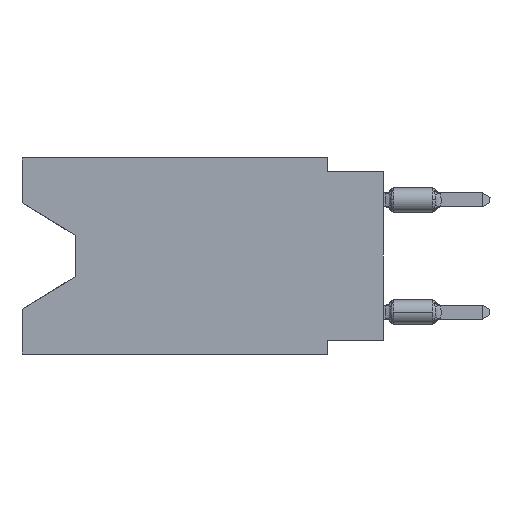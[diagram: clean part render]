
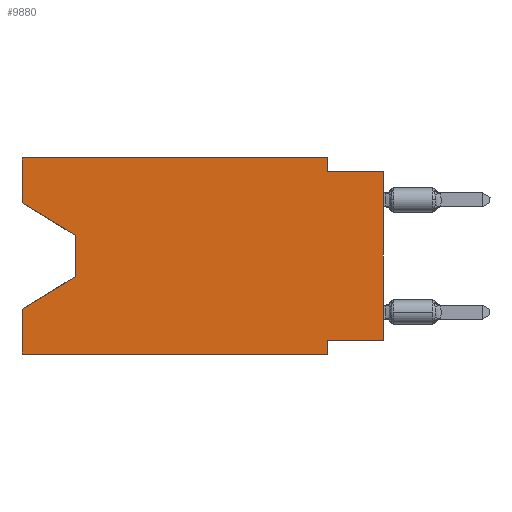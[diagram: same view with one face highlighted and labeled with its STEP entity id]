
A CAD part, left-side view. The second image highlights one B-rep face of the part: STEP entity #9880.
In plain terms, the highlighted planar face has unit normal (-1, 0, 0).
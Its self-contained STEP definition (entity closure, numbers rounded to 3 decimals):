
#218 = ORIENTED_EDGE ( 'NONE', *, *, #61031, .T. ) ;
#898 = LINE ( 'NONE', #48682, #18577 ) ;
#3849 = VERTEX_POINT ( 'NONE', #51764 ) ;
#3941 = CARTESIAN_POINT ( 'NONE',  ( 0., 13.97, -5.385 ) ) ;
#5513 = EDGE_CURVE ( 'NONE', #23257, #10101, #52324, .T. ) ;
#5767 = EDGE_CURVE ( 'NONE', #45476, #48817, #41096, .T. ) ;
#7909 = EDGE_CURVE ( 'NONE', #26975, #51505, #39138, .T. ) ;
#8350 = ORIENTED_EDGE ( 'NONE', *, *, #55840, .F. ) ;
#8451 = DIRECTION ( 'NONE',  ( 1., 0., 0. ) ) ;
#8663 = CARTESIAN_POINT ( 'NONE',  ( 0., 16.383, 0. ) ) ;
#8837 = CARTESIAN_POINT ( 'NONE',  ( 0., 16.383, 0. ) ) ;
#9020 = VECTOR ( 'NONE', #38017, 1000. ) ;
#9143 = DIRECTION ( 'NONE',  ( 0., -0.855, -0.519 ) ) ;
#9880 = ADVANCED_FACE ( 'NONE', ( #23721 ), #57855, .F. ) ;
#10101 = VERTEX_POINT ( 'NONE', #12437 ) ;
#10320 = LINE ( 'NONE', #8837, #57527 ) ;
#10482 = EDGE_LOOP ( 'NONE', ( #36207, #53071, #25910, #8350, #218, #14693, #40935, #35727, #20736, #42518, #43916, #48797 ) ) ;
#10778 = DIRECTION ( 'NONE',  ( 0., -1., 0. ) ) ;
#10949 = CARTESIAN_POINT ( 'NONE',  ( 0., 13.97, -5.385 ) ) ;
#11733 = VERTEX_POINT ( 'NONE', #34187 ) ;
#12019 = CARTESIAN_POINT ( 'NONE',  ( 0., 2.54, -8.89 ) ) ;
#12437 = CARTESIAN_POINT ( 'NONE',  ( 0., 16.383, 0. ) ) ;
#13182 = VECTOR ( 'NONE', #48444, 1000. ) ;
#14693 = ORIENTED_EDGE ( 'NONE', *, *, #51194, .F. ) ;
#15480 = VECTOR ( 'NONE', #26357, 1000. ) ;
#16600 = CARTESIAN_POINT ( 'NONE',  ( 0., 16.383, -8.89 ) ) ;
#17453 = VERTEX_POINT ( 'NONE', #34656 ) ;
#17732 = LINE ( 'NONE', #62361, #24379 ) ;
#17740 = VECTOR ( 'NONE', #61946, 1000. ) ;
#18225 = CARTESIAN_POINT ( 'NONE',  ( 0., 2.54, 0. ) ) ;
#18577 = VECTOR ( 'NONE', #33699, 1000. ) ;
#18623 = DIRECTION ( 'NONE',  ( 0., 0., -1. ) ) ;
#20293 = EDGE_CURVE ( 'NONE', #11733, #17453, #53243, .T. ) ;
#20736 = ORIENTED_EDGE ( 'NONE', *, *, #7909, .F. ) ;
#21251 = CARTESIAN_POINT ( 'NONE',  ( 0., 0., 0. ) ) ;
#21344 = DIRECTION ( 'NONE',  ( 0., 0., -1. ) ) ;
#21883 = LINE ( 'NONE', #21251, #15480 ) ;
#22812 = VERTEX_POINT ( 'NONE', #16600 ) ;
#23257 = VERTEX_POINT ( 'NONE', #51132 ) ;
#23378 = LINE ( 'NONE', #62272, #9020 ) ;
#23721 = FACE_OUTER_BOUND ( 'NONE', #10482, .T. ) ;
#24379 = VECTOR ( 'NONE', #9143, 1000. ) ;
#25910 = ORIENTED_EDGE ( 'NONE', *, *, #40899, .T. ) ;
#26357 = DIRECTION ( 'NONE',  ( 0., 0., 1. ) ) ;
#26975 = VERTEX_POINT ( 'NONE', #30110 ) ;
#27256 = CARTESIAN_POINT ( 'NONE',  ( 0., 2.54, -8.89 ) ) ;
#27773 = DIRECTION ( 'NONE',  ( 0., 0., 1. ) ) ;
#28382 = CARTESIAN_POINT ( 'NONE',  ( 0., 0., -8.255 ) ) ;
#29749 = DIRECTION ( 'NONE',  ( 0., -1., 0. ) ) ;
#30110 = CARTESIAN_POINT ( 'NONE',  ( 0., 2.54, -0.635 ) ) ;
#30791 = VERTEX_POINT ( 'NONE', #54090 ) ;
#31002 = VERTEX_POINT ( 'NONE', #27256 ) ;
#33081 = EDGE_CURVE ( 'NONE', #11733, #51505, #21883, .T. ) ;
#33699 = DIRECTION ( 'NONE',  ( 0., -1., 0. ) ) ;
#34187 = CARTESIAN_POINT ( 'NONE',  ( 0., 0., -8.255 ) ) ;
#34204 = VECTOR ( 'NONE', #27773, 1000. ) ;
#34656 = CARTESIAN_POINT ( 'NONE',  ( 0., 2.54, -8.255 ) ) ;
#35727 = ORIENTED_EDGE ( 'NONE', *, *, #33081, .T. ) ;
#36207 = ORIENTED_EDGE ( 'NONE', *, *, #56956, .T. ) ;
#37781 = LINE ( 'NONE', #12019, #40115 ) ;
#38017 = DIRECTION ( 'NONE',  ( 0., 0., 1. ) ) ;
#39138 = LINE ( 'NONE', #39776, #58549 ) ;
#39776 = CARTESIAN_POINT ( 'NONE',  ( 0., 0., -0.635 ) ) ;
#40115 = VECTOR ( 'NONE', #52149, 1000. ) ;
#40899 = EDGE_CURVE ( 'NONE', #48817, #3849, #52061, .T. ) ;
#40935 = ORIENTED_EDGE ( 'NONE', *, *, #20293, .F. ) ;
#41096 = LINE ( 'NONE', #59633, #48544 ) ;
#41191 = LINE ( 'NONE', #18225, #51647 ) ;
#42518 = ORIENTED_EDGE ( 'NONE', *, *, #54410, .F. ) ;
#43038 = CARTESIAN_POINT ( 'NONE',  ( 0., 0., -0.635 ) ) ;
#43349 = AXIS2_PLACEMENT_3D ( 'NONE', #52112, #8451, #18623 ) ;
#43916 = ORIENTED_EDGE ( 'NONE', *, *, #49964, .F. ) ;
#45476 = VERTEX_POINT ( 'NONE', #52864 ) ;
#48444 = DIRECTION ( 'NONE',  ( 0., 1., 0. ) ) ;
#48544 = VECTOR ( 'NONE', #21344, 1000. ) ;
#48682 = CARTESIAN_POINT ( 'NONE',  ( 0., 16.383, -8.89 ) ) ;
#48797 = ORIENTED_EDGE ( 'NONE', *, *, #5513, .F. ) ;
#48817 = VERTEX_POINT ( 'NONE', #10949 ) ;
#49964 = EDGE_CURVE ( 'NONE', #10101, #30791, #10320, .T. ) ;
#51132 = CARTESIAN_POINT ( 'NONE',  ( 0., 16.383, -2.038 ) ) ;
#51194 = EDGE_CURVE ( 'NONE', #17453, #31002, #37781, .T. ) ;
#51505 = VERTEX_POINT ( 'NONE', #43038 ) ;
#51647 = VECTOR ( 'NONE', #61293, 1000. ) ;
#51764 = CARTESIAN_POINT ( 'NONE',  ( 0., 16.383, -6.852 ) ) ;
#52061 = LINE ( 'NONE', #3941, #17740 ) ;
#52112 = CARTESIAN_POINT ( 'NONE',  ( 0., 16.383, 0. ) ) ;
#52149 = DIRECTION ( 'NONE',  ( 0., 0., -1. ) ) ;
#52324 = LINE ( 'NONE', #8663, #34204 ) ;
#52864 = CARTESIAN_POINT ( 'NONE',  ( 0., 13.97, -3.505 ) ) ;
#53071 = ORIENTED_EDGE ( 'NONE', *, *, #5767, .T. ) ;
#53243 = LINE ( 'NONE', #28382, #13182 ) ;
#54090 = CARTESIAN_POINT ( 'NONE',  ( 0., 2.54, 0. ) ) ;
#54410 = EDGE_CURVE ( 'NONE', #30791, #26975, #41191, .T. ) ;
#55840 = EDGE_CURVE ( 'NONE', #22812, #3849, #23378, .T. ) ;
#56956 = EDGE_CURVE ( 'NONE', #23257, #45476, #17732, .T. ) ;
#57527 = VECTOR ( 'NONE', #29749, 1000. ) ;
#57855 = PLANE ( 'NONE',  #43349 ) ;
#58549 = VECTOR ( 'NONE', #10778, 1000. ) ;
#59633 = CARTESIAN_POINT ( 'NONE',  ( 0., 13.97, -3.505 ) ) ;
#61031 = EDGE_CURVE ( 'NONE', #22812, #31002, #898, .T. ) ;
#61293 = DIRECTION ( 'NONE',  ( 0., 0., -1. ) ) ;
#61946 = DIRECTION ( 'NONE',  ( 0., 0.855, -0.519 ) ) ;
#62272 = CARTESIAN_POINT ( 'NONE',  ( 0., 16.383, 0. ) ) ;
#62361 = CARTESIAN_POINT ( 'NONE',  ( 0., 16.383, -2.038 ) ) ;
